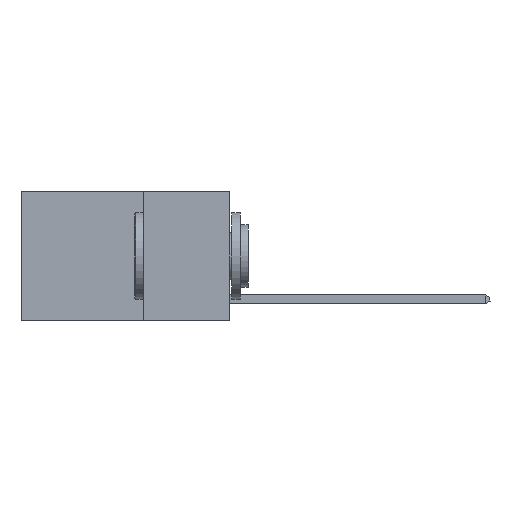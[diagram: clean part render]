
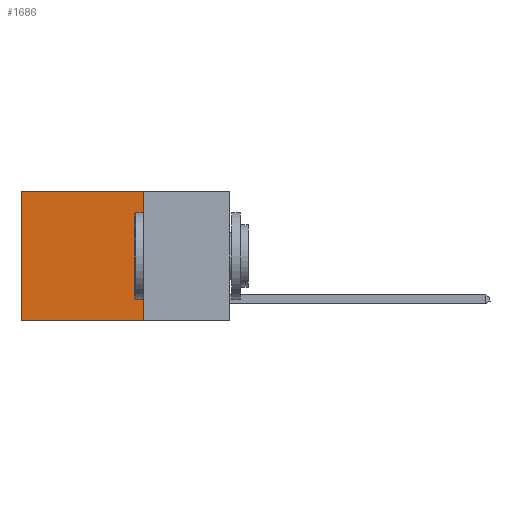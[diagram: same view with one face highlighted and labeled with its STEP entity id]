
A CAD part, left-side view. The second image highlights one B-rep face of the part: STEP entity #1686.
In plain terms, the highlighted planar face has unit normal (-1, 0, 0).
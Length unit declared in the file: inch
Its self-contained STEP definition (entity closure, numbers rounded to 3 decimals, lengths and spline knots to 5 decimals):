
#619 = VERTEX_POINT ( 'NONE', #11398 ) ;
#1463 = LINE ( 'NONE', #16435, #8508 ) ;
#1686 = ADVANCED_FACE ( 'NONE', ( #5310 ), #5502, .F. ) ;
#1893 = LINE ( 'NONE', #14230, #3769 ) ;
#2054 = ORIENTED_EDGE ( 'NONE', *, *, #6310, .F. ) ;
#2945 = DIRECTION ( 'NONE',  ( 1., 0., 0. ) ) ;
#2976 = LINE ( 'NONE', #3069, #7904 ) ;
#3069 = CARTESIAN_POINT ( 'NONE',  ( 0.2625, 0.25, 0. ) ) ;
#3769 = VECTOR ( 'NONE', #11504, 39.37008 ) ;
#4717 = VERTEX_POINT ( 'NONE', #12493 ) ;
#4881 = ORIENTED_EDGE ( 'NONE', *, *, #17741, .F. ) ;
#5310 = FACE_OUTER_BOUND ( 'NONE', #10355, .T. ) ;
#5502 = PLANE ( 'NONE',  #8648 ) ;
#6310 = EDGE_CURVE ( 'NONE', #4717, #619, #1463, .T. ) ;
#6524 = EDGE_CURVE ( 'NONE', #17655, #619, #10236, .T. ) ;
#7904 = VECTOR ( 'NONE', #8703, 39.37008 ) ;
#8248 = CARTESIAN_POINT ( 'NONE',  ( 0.2625, 0.25, 0. ) ) ;
#8508 = VECTOR ( 'NONE', #9697, 39.37008 ) ;
#8642 = CARTESIAN_POINT ( 'NONE',  ( 0.2625, 0.25, 0. ) ) ;
#8648 = AXIS2_PLACEMENT_3D ( 'NONE', #8248, #2945, #15239 ) ;
#8703 = DIRECTION ( 'NONE',  ( 0., 0., -1. ) ) ;
#9697 = DIRECTION ( 'NONE',  ( 0., 1., 0. ) ) ;
#9764 = ORIENTED_EDGE ( 'NONE', *, *, #13159, .T. ) ;
#9962 = CARTESIAN_POINT ( 'NONE',  ( 0.2625, 0.6, 0. ) ) ;
#10236 = LINE ( 'NONE', #9962, #12568 ) ;
#10355 = EDGE_LOOP ( 'NONE', ( #15609, #2054, #4881, #9764 ) ) ;
#11023 = VERTEX_POINT ( 'NONE', #8642 ) ;
#11398 = CARTESIAN_POINT ( 'NONE',  ( 0.2625, 0.6, -0.37 ) ) ;
#11504 = DIRECTION ( 'NONE',  ( 0., 1., 0. ) ) ;
#12493 = CARTESIAN_POINT ( 'NONE',  ( 0.2625, 0.25, -0.37 ) ) ;
#12568 = VECTOR ( 'NONE', #17066, 39.37008 ) ;
#12705 = CARTESIAN_POINT ( 'NONE',  ( 0.2625, 0.6, 0. ) ) ;
#13159 = EDGE_CURVE ( 'NONE', #11023, #17655, #1893, .T. ) ;
#14230 = CARTESIAN_POINT ( 'NONE',  ( 0.2625, 0.25, 0. ) ) ;
#15239 = DIRECTION ( 'NONE',  ( 0., 0., -1. ) ) ;
#15609 = ORIENTED_EDGE ( 'NONE', *, *, #6524, .T. ) ;
#16435 = CARTESIAN_POINT ( 'NONE',  ( 0.2625, 0.25, -0.37 ) ) ;
#17066 = DIRECTION ( 'NONE',  ( 0., 0., -1. ) ) ;
#17655 = VERTEX_POINT ( 'NONE', #12705 ) ;
#17741 = EDGE_CURVE ( 'NONE', #11023, #4717, #2976, .T. ) ;
